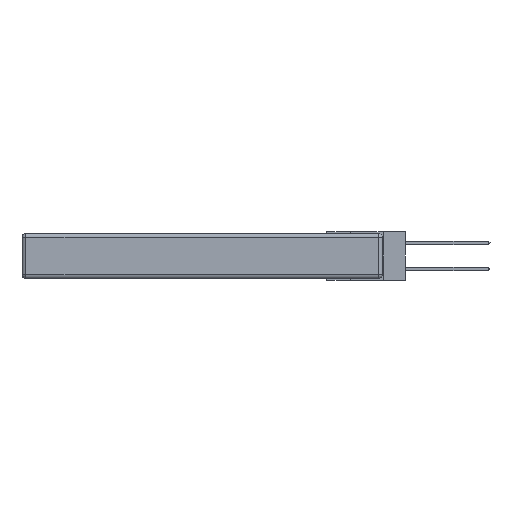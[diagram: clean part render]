
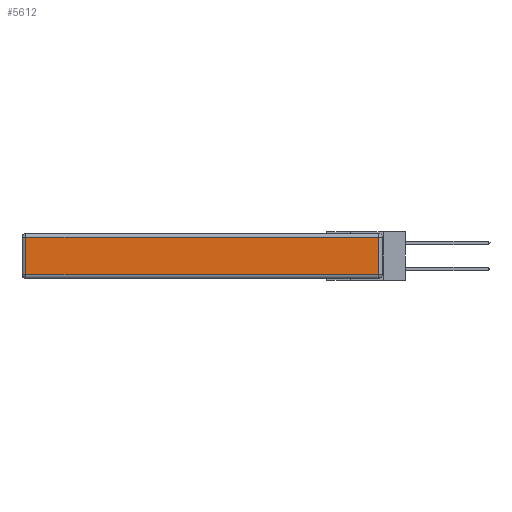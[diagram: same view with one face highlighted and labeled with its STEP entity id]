
A CAD part, left-side view. The second image highlights one B-rep face of the part: STEP entity #5612.
In plain terms, the highlighted planar face has unit normal (-1, 0, 0).
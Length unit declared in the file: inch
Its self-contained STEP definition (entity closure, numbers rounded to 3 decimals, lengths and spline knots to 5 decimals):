
#368 = EDGE_CURVE ( 'NONE', #8752, #12421, #7153, .T. ) ;
#422 = DIRECTION ( 'NONE',  ( 0., -1., 0. ) ) ;
#1129 = DIRECTION ( 'NONE',  ( 0., 0., -1. ) ) ;
#1597 = DIRECTION ( 'NONE',  ( 0., 1., 0. ) ) ;
#1936 = DIRECTION ( 'NONE',  ( -1., 0., 0. ) ) ;
#1949 = CARTESIAN_POINT ( 'NONE',  ( 0., 2.72, -0.03 ) ) ;
#2416 = VECTOR ( 'NONE', #422, 39.37008 ) ;
#3249 = DIRECTION ( 'NONE',  ( 0., 0., 1. ) ) ;
#4380 = CARTESIAN_POINT ( 'NONE',  ( 0., 0., -0.343 ) ) ;
#4996 = EDGE_LOOP ( 'NONE', ( #8360, #5724, #12452, #14166 ) ) ;
#5612 = ADVANCED_FACE ( 'NONE', ( #9109 ), #6933, .T. ) ;
#5724 = ORIENTED_EDGE ( 'NONE', *, *, #368, .T. ) ;
#6081 = VERTEX_POINT ( 'NONE', #7326 ) ;
#6113 = CARTESIAN_POINT ( 'NONE',  ( 0., 0.03, -0.313 ) ) ;
#6930 = LINE ( 'NONE', #15283, #14919 ) ;
#6933 = PLANE ( 'NONE',  #14682 ) ;
#7043 = EDGE_CURVE ( 'NONE', #12421, #9577, #6930, .T. ) ;
#7153 = LINE ( 'NONE', #12593, #14148 ) ;
#7209 = CARTESIAN_POINT ( 'NONE',  ( 0., 2.72, -0.343 ) ) ;
#7326 = CARTESIAN_POINT ( 'NONE',  ( 0., 2.72, -0.313 ) ) ;
#7613 = CARTESIAN_POINT ( 'NONE',  ( 0., 0.03, -0.03 ) ) ;
#8360 = ORIENTED_EDGE ( 'NONE', *, *, #8925, .T. ) ;
#8752 = VERTEX_POINT ( 'NONE', #6113 ) ;
#8925 = EDGE_CURVE ( 'NONE', #6081, #8752, #15828, .T. ) ;
#9109 = FACE_OUTER_BOUND ( 'NONE', #4996, .T. ) ;
#9577 = VERTEX_POINT ( 'NONE', #1949 ) ;
#10009 = VECTOR ( 'NONE', #1129, 39.37008 ) ;
#10021 = DIRECTION ( 'NONE',  ( 0., 0., 1. ) ) ;
#11282 = EDGE_CURVE ( 'NONE', #9577, #6081, #12341, .T. ) ;
#11362 = CARTESIAN_POINT ( 'NONE',  ( 0., 0., -0.313 ) ) ;
#12341 = LINE ( 'NONE', #7209, #10009 ) ;
#12421 = VERTEX_POINT ( 'NONE', #7613 ) ;
#12452 = ORIENTED_EDGE ( 'NONE', *, *, #7043, .T. ) ;
#12593 = CARTESIAN_POINT ( 'NONE',  ( 0., 0.03, -0.343 ) ) ;
#14148 = VECTOR ( 'NONE', #10021, 39.37008 ) ;
#14166 = ORIENTED_EDGE ( 'NONE', *, *, #11282, .T. ) ;
#14682 = AXIS2_PLACEMENT_3D ( 'NONE', #4380, #1936, #3249 ) ;
#14919 = VECTOR ( 'NONE', #1597, 39.37008 ) ;
#15283 = CARTESIAN_POINT ( 'NONE',  ( 0., 2.75, -0.03 ) ) ;
#15828 = LINE ( 'NONE', #11362, #2416 ) ;
